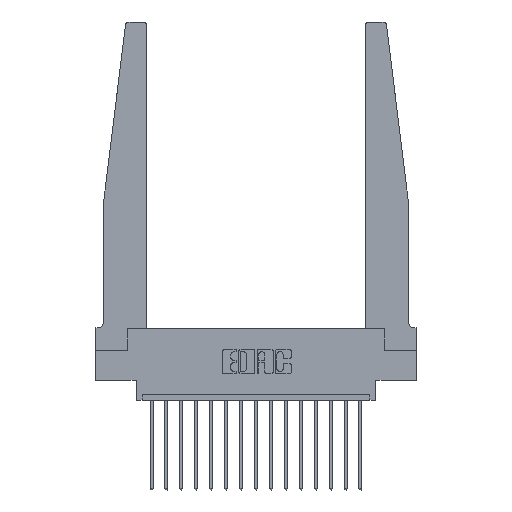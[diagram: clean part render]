
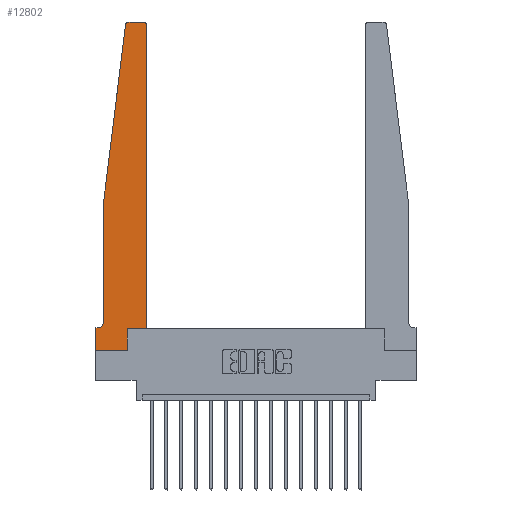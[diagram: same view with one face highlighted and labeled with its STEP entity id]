
A CAD part, top view. The second image highlights one B-rep face of the part: STEP entity #12802.
In plain terms, the highlighted planar face has unit normal (0, 0, 1).
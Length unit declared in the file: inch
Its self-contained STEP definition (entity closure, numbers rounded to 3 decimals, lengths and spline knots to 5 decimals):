
#190 = CIRCLE ( 'NONE', #7290, 0.05 ) ;
#560 = ORIENTED_EDGE ( 'NONE', *, *, #10879, .T. ) ;
#910 = EDGE_CURVE ( 'NONE', #4129, #5829, #4146, .T. ) ;
#933 = AXIS2_PLACEMENT_3D ( 'NONE', #1876, #3173, #8823 ) ;
#1098 = ORIENTED_EDGE ( 'NONE', *, *, #9222, .T. ) ;
#1170 = CARTESIAN_POINT ( 'NONE',  ( 0.2605, 0.18, 0.37 ) ) ;
#1326 = CARTESIAN_POINT ( 'NONE',  ( 0., 0.1875, 0.37 ) ) ;
#1453 = CARTESIAN_POINT ( 'NONE',  ( 0.395, 2.75, 0.37 ) ) ;
#1624 = VECTOR ( 'NONE', #15129, 39.37008 ) ;
#1644 = DIRECTION ( 'NONE',  ( -0.122, -0.992, 0. ) ) ;
#1703 = EDGE_CURVE ( 'NONE', #17981, #10152, #13548, .T. ) ;
#1803 = EDGE_CURVE ( 'NONE', #8820, #8932, #3217, .T. ) ;
#1876 = CARTESIAN_POINT ( 'NONE',  ( 0.27653, 2.72, 0.37 ) ) ;
#2245 = DIRECTION ( 'NONE',  ( -1., 0., 0. ) ) ;
#2387 = ORIENTED_EDGE ( 'NONE', *, *, #910, .T. ) ;
#2441 = CARTESIAN_POINT ( 'NONE',  ( 0.065, 0.2375, 0.37 ) ) ;
#3173 = DIRECTION ( 'NONE',  ( 0., 0., 1. ) ) ;
#3217 = LINE ( 'NONE', #11639, #9439 ) ;
#3234 = DIRECTION ( 'NONE',  ( 1., 0., 0. ) ) ;
#3510 = FACE_OUTER_BOUND ( 'NONE', #16358, .T. ) ;
#3888 = ORIENTED_EDGE ( 'NONE', *, *, #8853, .T. ) ;
#4129 = VERTEX_POINT ( 'NONE', #1326 ) ;
#4146 = LINE ( 'NONE', #7275, #5937 ) ;
#4286 = VECTOR ( 'NONE', #8497, 39.37008 ) ;
#4364 = DIRECTION ( 'NONE',  ( 0., 0., 1. ) ) ;
#4596 = CARTESIAN_POINT ( 'NONE',  ( 0.425, 0.18, 0.37 ) ) ;
#4730 = VERTEX_POINT ( 'NONE', #1170 ) ;
#4788 = DIRECTION ( 'NONE',  ( -1., 0., 0. ) ) ;
#4820 = EDGE_CURVE ( 'NONE', #16360, #4129, #11624, .T. ) ;
#4967 = CARTESIAN_POINT ( 'NONE',  ( 0.015, 0.2375, 0.37 ) ) ;
#5121 = EDGE_CURVE ( 'NONE', #7701, #4730, #15362, .T. ) ;
#5207 = VERTEX_POINT ( 'NONE', #2441 ) ;
#5364 = ORIENTED_EDGE ( 'NONE', *, *, #6850, .T. ) ;
#5829 = VERTEX_POINT ( 'NONE', #14776 ) ;
#5937 = VECTOR ( 'NONE', #10032, 39.37008 ) ;
#5942 = CARTESIAN_POINT ( 'NONE',  ( 0.425, 0.18, 0.37 ) ) ;
#6128 = PLANE ( 'NONE',  #8544 ) ;
#6628 = LINE ( 'NONE', #10581, #16053 ) ;
#6850 = EDGE_CURVE ( 'NONE', #5207, #16360, #190, .T. ) ;
#7275 = CARTESIAN_POINT ( 'NONE',  ( 0., 0., 0.37 ) ) ;
#7290 = AXIS2_PLACEMENT_3D ( 'NONE', #4967, #10571, #4788 ) ;
#7379 = DIRECTION ( 'NONE',  ( 1., 0., 0. ) ) ;
#7701 = VERTEX_POINT ( 'NONE', #17357 ) ;
#8234 = LINE ( 'NONE', #11090, #12849 ) ;
#8424 = DIRECTION ( 'NONE',  ( 0., -1., 0. ) ) ;
#8497 = DIRECTION ( 'NONE',  ( -1., 0., 0. ) ) ;
#8521 = VECTOR ( 'NONE', #12444, 39.37008 ) ;
#8544 = AXIS2_PLACEMENT_3D ( 'NONE', #9247, #10350, #3234 ) ;
#8704 = EDGE_CURVE ( 'NONE', #5829, #7701, #9165, .T. ) ;
#8806 = ORIENTED_EDGE ( 'NONE', *, *, #1803, .T. ) ;
#8820 = VERTEX_POINT ( 'NONE', #16166 ) ;
#8823 = DIRECTION ( 'NONE',  ( 1., 0., 0. ) ) ;
#8853 = EDGE_CURVE ( 'NONE', #8932, #5207, #8234, .T. ) ;
#8932 = VERTEX_POINT ( 'NONE', #18293 ) ;
#9165 = LINE ( 'NONE', #12097, #1624 ) ;
#9219 = CIRCLE ( 'NONE', #933, 0.03 ) ;
#9222 = EDGE_CURVE ( 'NONE', #11932, #17981, #11906, .T. ) ;
#9247 = CARTESIAN_POINT ( 'NONE',  ( 0., 0.1875, 0.37 ) ) ;
#9439 = VECTOR ( 'NONE', #1644, 39.37008 ) ;
#9495 = CARTESIAN_POINT ( 'NONE',  ( 0.425, 0.18, 0.37 ) ) ;
#9582 = VECTOR ( 'NONE', #17163, 39.37008 ) ;
#9720 = AXIS2_PLACEMENT_3D ( 'NONE', #14207, #4364, #7379 ) ;
#9740 = CARTESIAN_POINT ( 'NONE',  ( 0.27653, 2.75, 0.37 ) ) ;
#10032 = DIRECTION ( 'NONE',  ( 0., -1., 0. ) ) ;
#10152 = VERTEX_POINT ( 'NONE', #1453 ) ;
#10159 = VECTOR ( 'NONE', #13895, 39.37008 ) ;
#10271 = EDGE_CURVE ( 'NONE', #4730, #11932, #14381, .T. ) ;
#10350 = DIRECTION ( 'NONE',  ( 0., 0., 1. ) ) ;
#10545 = ORIENTED_EDGE ( 'NONE', *, *, #5121, .T. ) ;
#10571 = DIRECTION ( 'NONE',  ( 0., 0., -1. ) ) ;
#10581 = CARTESIAN_POINT ( 'NONE',  ( 0.25, 2.75, 0.37 ) ) ;
#10594 = EDGE_CURVE ( 'NONE', #10152, #14918, #6628, .T. ) ;
#10879 = EDGE_CURVE ( 'NONE', #14918, #8820, #9219, .T. ) ;
#11090 = CARTESIAN_POINT ( 'NONE',  ( 0.065, 1.25, 0.37 ) ) ;
#11419 = CARTESIAN_POINT ( 'NONE',  ( 0.015, 0.1875, 0.37 ) ) ;
#11624 = LINE ( 'NONE', #14092, #4286 ) ;
#11639 = CARTESIAN_POINT ( 'NONE',  ( 0.065, 1.25, 0.37 ) ) ;
#11906 = LINE ( 'NONE', #9495, #8521 ) ;
#11932 = VERTEX_POINT ( 'NONE', #4596 ) ;
#12097 = CARTESIAN_POINT ( 'NONE',  ( 0., 0., 0.37 ) ) ;
#12189 = ORIENTED_EDGE ( 'NONE', *, *, #10271, .T. ) ;
#12444 = DIRECTION ( 'NONE',  ( 0., 1., 0. ) ) ;
#12802 = ADVANCED_FACE ( 'NONE', ( #3510 ), #6128, .T. ) ;
#12849 = VECTOR ( 'NONE', #8424, 39.37008 ) ;
#13548 = CIRCLE ( 'NONE', #9720, 0.03 ) ;
#13895 = DIRECTION ( 'NONE',  ( 0., 1., 0. ) ) ;
#14071 = ORIENTED_EDGE ( 'NONE', *, *, #10594, .T. ) ;
#14092 = CARTESIAN_POINT ( 'NONE',  ( 0.065, 0.1875, 0.37 ) ) ;
#14207 = CARTESIAN_POINT ( 'NONE',  ( 0.395, 2.72, 0.37 ) ) ;
#14381 = LINE ( 'NONE', #5942, #9582 ) ;
#14776 = CARTESIAN_POINT ( 'NONE',  ( 0., 0., 0.37 ) ) ;
#14918 = VERTEX_POINT ( 'NONE', #9740 ) ;
#15129 = DIRECTION ( 'NONE',  ( 1., 0., 0. ) ) ;
#15315 = ORIENTED_EDGE ( 'NONE', *, *, #8704, .T. ) ;
#15362 = LINE ( 'NONE', #16484, #10159 ) ;
#15558 = CARTESIAN_POINT ( 'NONE',  ( 0.425, 2.72, 0.37 ) ) ;
#16053 = VECTOR ( 'NONE', #2245, 39.37008 ) ;
#16166 = CARTESIAN_POINT ( 'NONE',  ( 0.24675, 2.72367, 0.37 ) ) ;
#16358 = EDGE_LOOP ( 'NONE', ( #14071, #560, #8806, #3888, #5364, #17192, #2387, #15315, #10545, #12189, #1098, #16762 ) ) ;
#16360 = VERTEX_POINT ( 'NONE', #11419 ) ;
#16484 = CARTESIAN_POINT ( 'NONE',  ( 0.2605, 0.18, 0.37 ) ) ;
#16762 = ORIENTED_EDGE ( 'NONE', *, *, #1703, .T. ) ;
#17163 = DIRECTION ( 'NONE',  ( 1., 0., 0. ) ) ;
#17192 = ORIENTED_EDGE ( 'NONE', *, *, #4820, .T. ) ;
#17357 = CARTESIAN_POINT ( 'NONE',  ( 0.2605, 0., 0.37 ) ) ;
#17981 = VERTEX_POINT ( 'NONE', #15558 ) ;
#18293 = CARTESIAN_POINT ( 'NONE',  ( 0.065, 1.25, 0.37 ) ) ;
